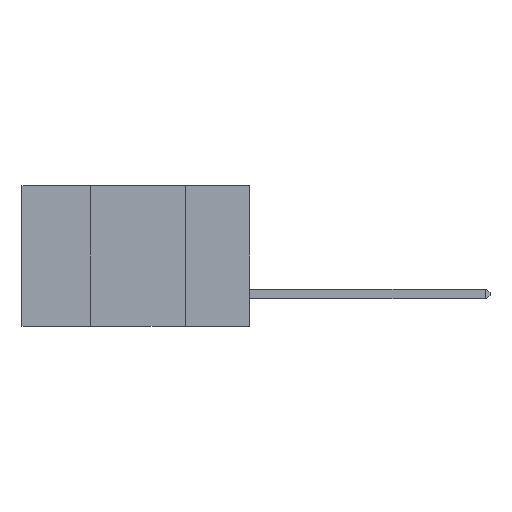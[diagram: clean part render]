
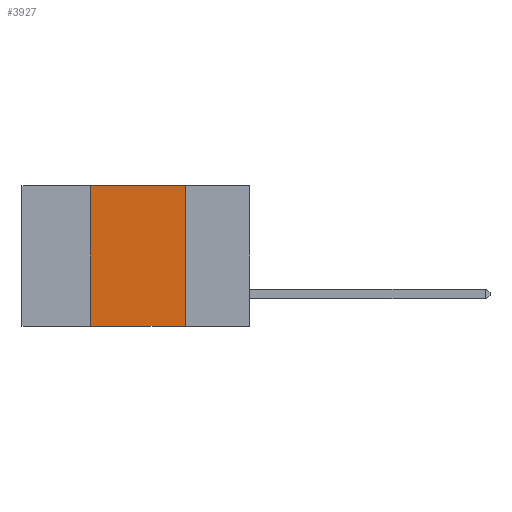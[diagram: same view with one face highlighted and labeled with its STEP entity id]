
A CAD part, left-side view. The second image highlights one B-rep face of the part: STEP entity #3927.
In plain terms, the highlighted planar face has unit normal (-1, 0, 0).
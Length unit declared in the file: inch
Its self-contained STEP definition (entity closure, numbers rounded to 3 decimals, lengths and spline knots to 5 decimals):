
#180 = VECTOR ( 'NONE', #2119, 39.37008 ) ;
#303 = ORIENTED_EDGE ( 'NONE', *, *, #3539, .F. ) ;
#413 = PLANE ( 'NONE',  #9777 ) ;
#477 = CARTESIAN_POINT ( 'NONE',  ( 0., 0.6, 0. ) ) ;
#695 = EDGE_CURVE ( 'NONE', #2209, #1701, #1039, .T. ) ;
#1039 = LINE ( 'NONE', #5322, #8992 ) ;
#1235 = ORIENTED_EDGE ( 'NONE', *, *, #3136, .T. ) ;
#1667 = EDGE_CURVE ( 'NONE', #9322, #2209, #2041, .T. ) ;
#1671 = CARTESIAN_POINT ( 'NONE',  ( 0., 0.17, 0. ) ) ;
#1701 = VERTEX_POINT ( 'NONE', #7900 ) ;
#2041 = LINE ( 'NONE', #8986, #6175 ) ;
#2119 = DIRECTION ( 'NONE',  ( 0., -1., 0. ) ) ;
#2209 = VERTEX_POINT ( 'NONE', #1671 ) ;
#2496 = DIRECTION ( 'NONE',  ( 0., -1., 0. ) ) ;
#2948 = ORIENTED_EDGE ( 'NONE', *, *, #695, .F. ) ;
#3136 = EDGE_CURVE ( 'NONE', #4167, #1701, #5201, .T. ) ;
#3539 = EDGE_CURVE ( 'NONE', #4167, #9322, #9282, .T. ) ;
#3824 = DIRECTION ( 'NONE',  ( 0., 0., -1. ) ) ;
#3882 = DIRECTION ( 'NONE',  ( 1., 0., 0. ) ) ;
#3927 = ADVANCED_FACE ( 'NONE', ( #5902 ), #413, .F. ) ;
#4070 = DIRECTION ( 'NONE',  ( 0., 0., -1. ) ) ;
#4167 = VERTEX_POINT ( 'NONE', #7166 ) ;
#5201 = LINE ( 'NONE', #7484, #180 ) ;
#5322 = CARTESIAN_POINT ( 'NONE',  ( 0., 0.17, 0. ) ) ;
#5902 = FACE_OUTER_BOUND ( 'NONE', #7689, .T. ) ;
#6175 = VECTOR ( 'NONE', #2496, 39.37008 ) ;
#6218 = DIRECTION ( 'NONE',  ( 0., 0., 1. ) ) ;
#7091 = CARTESIAN_POINT ( 'NONE',  ( 0., 0.42, 0. ) ) ;
#7166 = CARTESIAN_POINT ( 'NONE',  ( 0., 0.42, -0.37 ) ) ;
#7393 = VECTOR ( 'NONE', #6218, 39.37008 ) ;
#7484 = CARTESIAN_POINT ( 'NONE',  ( 0., 0.6, -0.37 ) ) ;
#7689 = EDGE_LOOP ( 'NONE', ( #2948, #7925, #303, #1235 ) ) ;
#7900 = CARTESIAN_POINT ( 'NONE',  ( 0., 0.17, -0.37 ) ) ;
#7925 = ORIENTED_EDGE ( 'NONE', *, *, #1667, .F. ) ;
#8986 = CARTESIAN_POINT ( 'NONE',  ( 0., 0.6, 0. ) ) ;
#8992 = VECTOR ( 'NONE', #4070, 39.37008 ) ;
#9282 = LINE ( 'NONE', #9360, #7393 ) ;
#9322 = VERTEX_POINT ( 'NONE', #7091 ) ;
#9360 = CARTESIAN_POINT ( 'NONE',  ( 0., 0.42, 0. ) ) ;
#9777 = AXIS2_PLACEMENT_3D ( 'NONE', #477, #3882, #3824 ) ;
